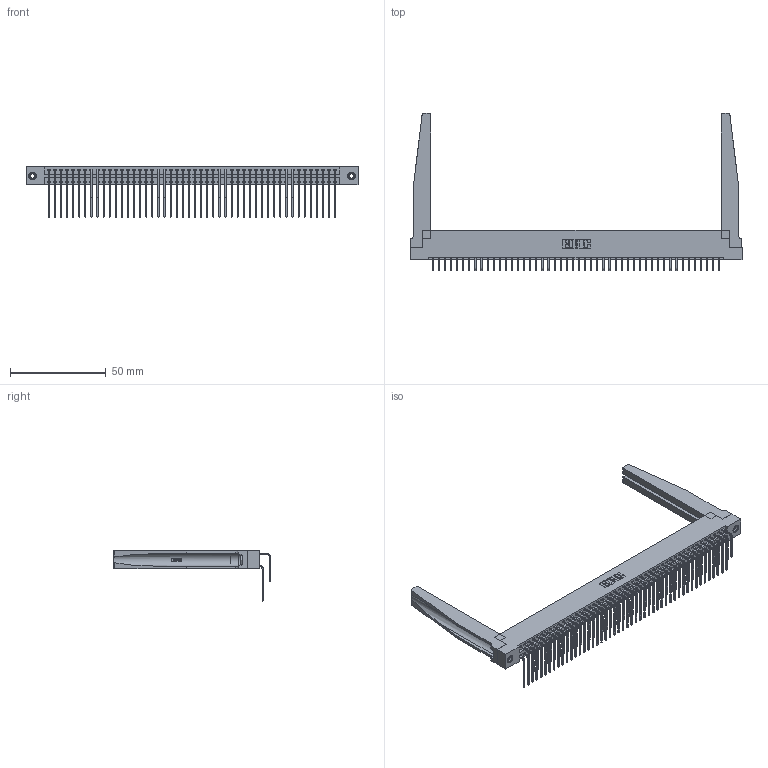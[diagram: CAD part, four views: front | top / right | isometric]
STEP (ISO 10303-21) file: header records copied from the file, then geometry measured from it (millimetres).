
FILE_DESCRIPTION (( 'STEP AP203' ), '1' );
FILE_NAME ('396-096-559-278.STEP', '2019-11-03T15:28:19', ( '' ), ( '' ), 'SwSTEP 2.0', 'SolidWorks 2016', '' );
FILE_SCHEMA (( 'CONFIG_CONTROL_DESIGN' ));
Length unit declared in the file: inch
Products named in the file (6): 396-096-559-278; 345-292-001_559 Tail - 2; 345-292-001_558 559 Tail - 1; 346-220-078_345-220-078; 345-250-001_345-250-001-102; 346 Part_Flush Mounting Lugs - 0.156 Dia-TH
Assembly tree (101 placements, depth 2):
  396-096-559-278
    346 Part_Flush Mounting Lugs - 0.156 Dia-TH
    345-292-001_558 559 Tail - 1  x48
    345-292-001_559 Tail - 2  x48
    346-220-078_345-220-078  x2
    345-250-001_345-250-001-102  x2
Bounding box: 172.97 x 81.85 x 26.16 mm (x, y, z)
Volume: 24376.4 mm3; surface area: 33298.9 mm2
Topology: 101 solids, 101 shells, 5540 faces, 16393 edges, 10790 vertices
Faces by surface type: plane 3770, cylinder 1718, bspline 36, cone 12, torus 4
Entity records: 37050 total; most frequent: CARTESIAN_POINT 7086, ORIENTED_EDGE 5858, DIRECTION 5255, EDGE_CURVE 2929, VECTOR 2471, LINE 2471, VERTEX_POINT 1944, AXIS2_PLACEMENT_3D 1392
